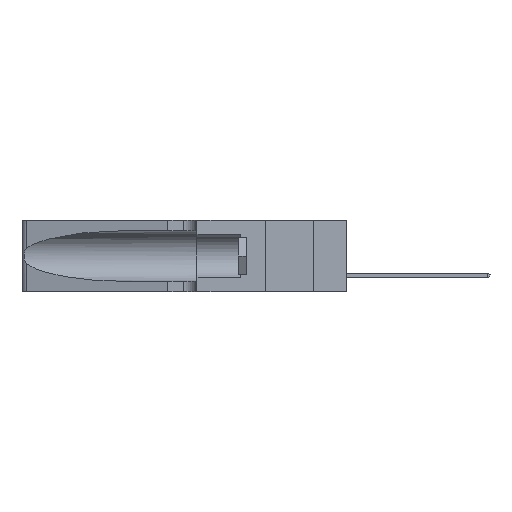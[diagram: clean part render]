
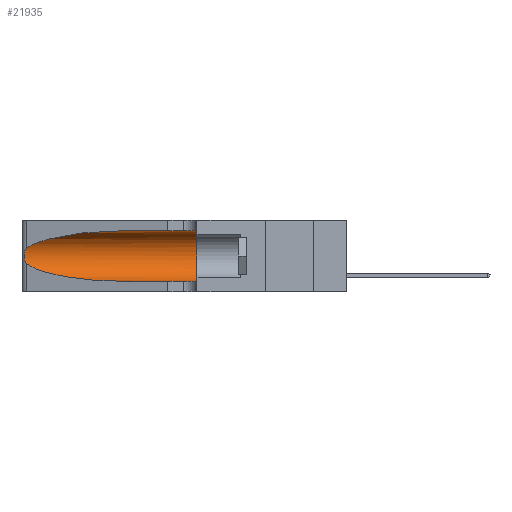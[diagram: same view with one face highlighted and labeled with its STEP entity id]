
A CAD part, left-side view. The second image highlights one B-rep face of the part: STEP entity #21935.
In plain terms, the highlighted cylindrical face has radius 3.308 mm (diameter 6.617 mm), a partial arc.
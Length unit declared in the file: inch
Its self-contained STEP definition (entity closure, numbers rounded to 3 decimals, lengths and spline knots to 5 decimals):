
#205 = CARTESIAN_POINT ( 'NONE',  ( 0.25487, 1.22718, 0.14631 ) ) ;
#497 = VERTEX_POINT ( 'NONE', #12641 ) ;
#1142 = CARTESIAN_POINT ( 'NONE',  ( 0.25487, 1.22718, 0.22369 ) ) ;
#2617 = VECTOR ( 'NONE', #32845, 39.37008 ) ;
#3250 = CARTESIAN_POINT ( 'NONE',  ( 0.1305, 0.72297, 0.05475 ) ) ;
#3580 = CARTESIAN_POINT ( 'NONE',  ( 0.1305, 1.61858, 0.05475 ) ) ;
#4149 = DIRECTION ( 'NONE',  ( 0., 1., 0. ) ) ;
#4300 = ORIENTED_EDGE ( 'NONE', *, *, #27814, .T. ) ;
#4449 = ORIENTED_EDGE ( 'NONE', *, *, #23749, .T. ) ;
#4638 = CARTESIAN_POINT ( 'NONE',  ( 0.1305, 0.35, 0.31525 ) ) ;
#6296 = CARTESIAN_POINT ( 'NONE',  ( 0.26017, 1.23833, 0.17102 ) ) ;
#6835 = ORIENTED_EDGE ( 'NONE', *, *, #18947, .F. ) ;
#6865 = DIRECTION ( 'NONE',  ( 0., 0., 1. ) ) ;
#9030 = CARTESIAN_POINT ( 'NONE',  ( 0.25856, 1.23593, 0.16098 ) ) ;
#9146 = CARTESIAN_POINT ( 'NONE',  ( 0.25639, 1.23184, 0.21858 ) ) ;
#9890 = CARTESIAN_POINT ( 'NONE',  ( 0.1305, 1.61858, 0.185 ) ) ;
#10558 = CARTESIAN_POINT ( 'NONE',  ( 0.18966, 0.96281, 0.31525 ) ) ;
#11755 = CARTESIAN_POINT ( 'NONE',  ( 0.25789, 1.23486, 0.15765 ) ) ;
#11998 = CARTESIAN_POINT ( 'NONE',  ( 0.26075, 1.23896, 0.19203 ) ) ;
#12641 = CARTESIAN_POINT ( 'NONE',  ( 0.25487, 1.22718, 0.14631 ) ) ;
#12794 = CARTESIAN_POINT ( 'NONE',  ( 0.25487, 1.22718, 0.22369 ) ) ;
#12800 = CARTESIAN_POINT ( 'NONE',  ( 0.1305, 1.61858, 0.31525 ) ) ;
#13336 = VERTEX_POINT ( 'NONE', #4638 ) ;
#13794 = CARTESIAN_POINT ( 'NONE',  ( 0.2373, 1.15595, 0.08982 ) ) ;
#14332 = EDGE_CURVE ( 'NONE', #23076, #13336, #19260, .T. ) ;
#14836 =( BOUNDED_CURVE ( )  B_SPLINE_CURVE ( 3, ( #205, #13794, #27990, #3250 ),
 .UNSPECIFIED., .F., .F. ) 
 B_SPLINE_CURVE_WITH_KNOTS ( ( 4, 4 ),
 ( 3.44316, 4.71239 ),
 .UNSPECIFIED. ) 
 CURVE ( )  GEOMETRIC_REPRESENTATION_ITEM ( )  RATIONAL_B_SPLINE_CURVE ( ( 1., 0.87, 0.87, 1. ) ) 
 REPRESENTATION_ITEM ( '' )  );
#14956 = CARTESIAN_POINT ( 'NONE',  ( 0.25555, 1.22994, 0.2215 ) ) ;
#18053 = EDGE_CURVE ( 'NONE', #33498, #26455, #34291, .T. ) ;
#18947 = EDGE_CURVE ( 'NONE', #13336, #26455, #23710, .T. ) ;
#19081 = CARTESIAN_POINT ( 'NONE',  ( 0.1305, 0.72297, 0.31525 ) ) ;
#19260 = LINE ( 'NONE', #12800, #30665 ) ;
#19926 = CARTESIAN_POINT ( 'NONE',  ( 0.25487, 1.22718, 0.14631 ) ) ;
#20176 = CARTESIAN_POINT ( 'NONE',  ( 0.26075, 1.23896, 0.178 ) ) ;
#20446 = ORIENTED_EDGE ( 'NONE', *, *, #22762, .T. ) ;
#21264 = FACE_OUTER_BOUND ( 'NONE', #27032, .T. ) ;
#21789 = AXIS2_PLACEMENT_3D ( 'NONE', #9890, #28701, #34400 ) ;
#21794 = CARTESIAN_POINT ( 'NONE',  ( 0.25487, 1.22718, 0.22369 ) ) ;
#21935 = ADVANCED_FACE ( 'NONE', ( #21264 ), #32194, .F. ) ;
#22200 = VERTEX_POINT ( 'NONE', #12794 ) ;
#22525 = CARTESIAN_POINT ( 'NONE',  ( 0.26018, 1.23835, 0.19895 ) ) ;
#22762 = EDGE_CURVE ( 'NONE', #22200, #497, #34696, .T. ) ;
#22972 = CARTESIAN_POINT ( 'NONE',  ( 0.1305, 0.35, 0.185 ) ) ;
#23076 = VERTEX_POINT ( 'NONE', #32972 ) ;
#23710 = CIRCLE ( 'NONE', #25578, 0.13025 ) ;
#23749 = EDGE_CURVE ( 'NONE', #497, #33498, #14836, .T. ) ;
#23895 = ORIENTED_EDGE ( 'NONE', *, *, #14332, .F. ) ;
#25578 = AXIS2_PLACEMENT_3D ( 'NONE', #22972, #4149, #6865 ) ;
#25584 = CARTESIAN_POINT ( 'NONE',  ( 0.1305, 0.35, 0.05475 ) ) ;
#26354 = CARTESIAN_POINT ( 'NONE',  ( 0.1305, 0.72297, 0.05475 ) ) ;
#26455 = VERTEX_POINT ( 'NONE', #25584 ) ;
#26511 = ORIENTED_EDGE ( 'NONE', *, *, #18053, .T. ) ;
#26752 =( BOUNDED_CURVE ( )  B_SPLINE_CURVE ( 3, ( #19081, #10558, #29718, #21794 ),
 .UNSPECIFIED., .F., .F. ) 
 B_SPLINE_CURVE_WITH_KNOTS ( ( 4, 4 ),
 ( 1.5708, 2.84003 ),
 .UNSPECIFIED. ) 
 CURVE ( )  GEOMETRIC_REPRESENTATION_ITEM ( )  RATIONAL_B_SPLINE_CURVE ( ( 1., 0.87, 0.87, 1. ) ) 
 REPRESENTATION_ITEM ( '' )  );
#27032 = EDGE_LOOP ( 'NONE', ( #4300, #20446, #4449, #26511, #6835, #23895 ) ) ;
#27814 = EDGE_CURVE ( 'NONE', #23076, #22200, #26752, .T. ) ;
#27990 = CARTESIAN_POINT ( 'NONE',  ( 0.18966, 0.96281, 0.05475 ) ) ;
#28086 = CARTESIAN_POINT ( 'NONE',  ( 0.25639, 1.23186, 0.15144 ) ) ;
#28701 = DIRECTION ( 'NONE',  ( 0., -1., 0. ) ) ;
#29175 = DIRECTION ( 'NONE',  ( 0., -1., 0. ) ) ;
#29718 = CARTESIAN_POINT ( 'NONE',  ( 0.2373, 1.15595, 0.28018 ) ) ;
#30665 = VECTOR ( 'NONE', #29175, 39.37008 ) ;
#30687 = CARTESIAN_POINT ( 'NONE',  ( 0.25555, 1.22993, 0.14849 ) ) ;
#32194 = CYLINDRICAL_SURFACE ( 'NONE', #21789, 0.13025 ) ;
#32845 = DIRECTION ( 'NONE',  ( 0., -1., 0. ) ) ;
#32972 = CARTESIAN_POINT ( 'NONE',  ( 0.1305, 0.72297, 0.31525 ) ) ;
#33339 = CARTESIAN_POINT ( 'NONE',  ( 0.25854, 1.2359, 0.20912 ) ) ;
#33454 = CARTESIAN_POINT ( 'NONE',  ( 0.25787, 1.23484, 0.2124 ) ) ;
#33498 = VERTEX_POINT ( 'NONE', #26354 ) ;
#34291 = LINE ( 'NONE', #3580, #2617 ) ;
#34400 = DIRECTION ( 'NONE',  ( 0., 0., -1. ) ) ;
#34696 = B_SPLINE_CURVE_WITH_KNOTS ( 'NONE', 3,
 ( #1142, #14956, #9146, #33454, #33339, #22525, #11998, #20176, #6296, #9030, #11755, #28086, #30687, #19926 ),
 .UNSPECIFIED., .F., .F.,
 ( 4, 2, 2, 2, 2, 2, 4 ),
 ( 0., 0.00027, 0.00053, 0.00107, 0.0016, 0.00187, 0.00214 ),
 .UNSPECIFIED. ) ;
